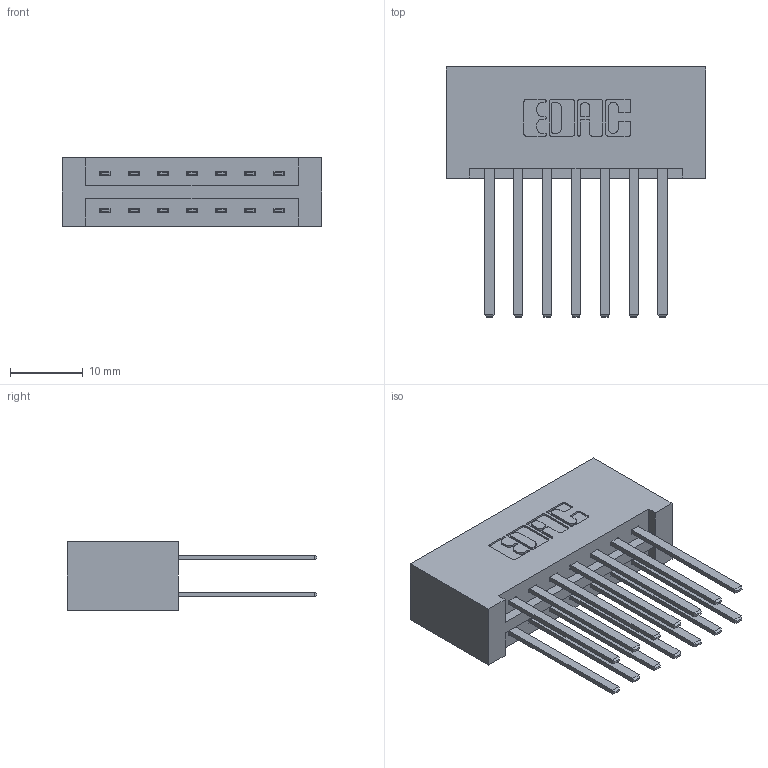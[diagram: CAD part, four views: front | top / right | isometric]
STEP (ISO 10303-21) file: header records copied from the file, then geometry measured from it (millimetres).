
FILE_DESCRIPTION (( 'STEP AP203' ), '1' );
FILE_NAME ('337-014-544-201.STEP', '2019-10-08T11:51:06', ( '' ), ( '' ), 'SwSTEP 2.0', 'SolidWorks 2016', '' );
FILE_SCHEMA (( 'CONFIG_CONTROL_DESIGN' ));
Length unit declared in the file: inch
Products named in the file (3): 337 Part_No Mounting Lugs; 345-292-001_345-293-144; 337-014-544-201
Assembly tree (15 placements, depth 2):
  337-014-544-201
    337 Part_No Mounting Lugs
    345-292-001_345-293-144  x14
Bounding box: 35.61 x 34.3 x 9.4 mm (x, y, z)
Volume: 4244.1 mm3; surface area: 5155.1 mm2
Topology: 15 solids, 15 shells, 778 faces, 2289 edges, 1506 vertices
Faces by surface type: plane 542, cylinder 236
Entity records: 9493 total; most frequent: CARTESIAN_POINT 1626, ORIENTED_EDGE 1562, DIRECTION 1437, EDGE_CURVE 781, LINE 665, VECTOR 665, VERTEX_POINT 518, AXIS2_PLACEMENT_3D 386
